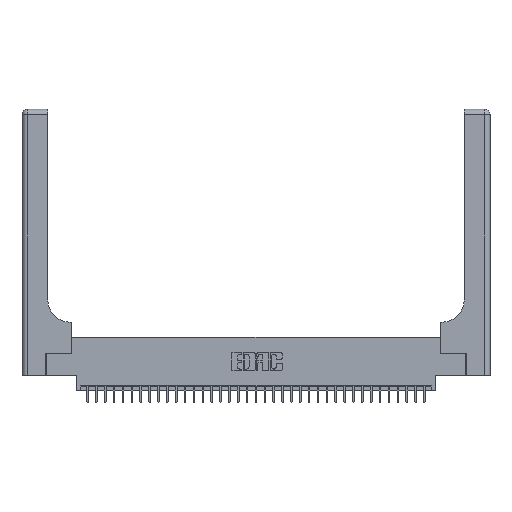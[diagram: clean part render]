
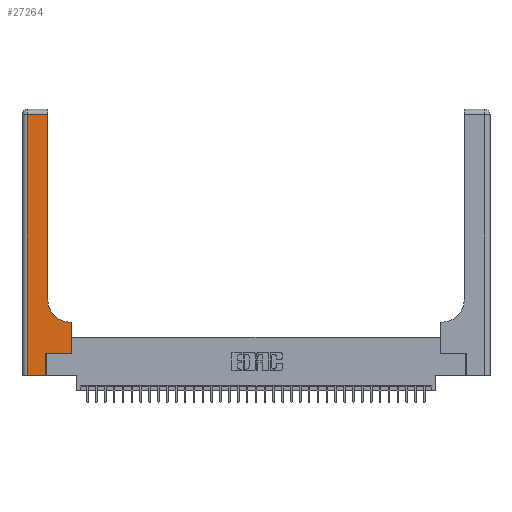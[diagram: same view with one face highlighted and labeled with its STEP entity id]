
A CAD part, top view. The second image highlights one B-rep face of the part: STEP entity #27264.
In plain terms, the highlighted planar face has unit normal (0, 0, 1).
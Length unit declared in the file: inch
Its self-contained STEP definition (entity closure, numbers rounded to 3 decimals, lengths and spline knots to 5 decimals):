
#1137 = ORIENTED_EDGE ( 'NONE', *, *, #33386, .T. ) ;
#1304 = DIRECTION ( 'NONE',  ( 0., 1., 0. ) ) ;
#1550 = ORIENTED_EDGE ( 'NONE', *, *, #27897, .T. ) ;
#2720 = CARTESIAN_POINT ( 'NONE',  ( 0.06, 3., 0.37 ) ) ;
#3202 = VERTEX_POINT ( 'NONE', #4219 ) ;
#3707 = DIRECTION ( 'NONE',  ( -1., 0., 0. ) ) ;
#4219 = CARTESIAN_POINT ( 'NONE',  ( 0.2915, 0.85, 0.37 ) ) ;
#4235 = LINE ( 'NONE', #32437, #14949 ) ;
#4299 = VECTOR ( 'NONE', #15855, 39.37008 ) ;
#4582 = CARTESIAN_POINT ( 'NONE',  ( 0., 3., 0.37 ) ) ;
#6160 = EDGE_LOOP ( 'NONE', ( #20468, #15500, #10927, #1550, #24159, #1137, #10253, #8115, #33073 ) ) ;
#6809 = PLANE ( 'NONE',  #35200 ) ;
#7383 = CARTESIAN_POINT ( 'NONE',  ( 0.269, 0., 0.37 ) ) ;
#8115 = ORIENTED_EDGE ( 'NONE', *, *, #22319, .T. ) ;
#8379 = DIRECTION ( 'NONE',  ( 1., 0., 0. ) ) ;
#8475 = VECTOR ( 'NONE', #31628, 39.37008 ) ;
#8681 = CARTESIAN_POINT ( 'NONE',  ( 0.2915, 3., 0.37 ) ) ;
#8790 = CARTESIAN_POINT ( 'NONE',  ( 0.2915, 0.6, 0.37 ) ) ;
#8953 = EDGE_CURVE ( 'NONE', #3202, #18350, #30642, .T. ) ;
#9272 = CARTESIAN_POINT ( 'NONE',  ( 0.269, 0.25, 0.37 ) ) ;
#9413 = CARTESIAN_POINT ( 'NONE',  ( 0., 0., 0.37 ) ) ;
#9962 = CARTESIAN_POINT ( 'NONE',  ( 0.5415, 0.6, 0.37 ) ) ;
#10114 = DIRECTION ( 'NONE',  ( 0., 0., -1. ) ) ;
#10167 = LINE ( 'NONE', #21413, #4299 ) ;
#10253 = ORIENTED_EDGE ( 'NONE', *, *, #17465, .T. ) ;
#10927 = ORIENTED_EDGE ( 'NONE', *, *, #33637, .T. ) ;
#11437 = CARTESIAN_POINT ( 'NONE',  ( 0., 2.94, 0.37 ) ) ;
#11893 = VERTEX_POINT ( 'NONE', #28991 ) ;
#12168 = LINE ( 'NONE', #9413, #22862 ) ;
#12413 = VERTEX_POINT ( 'NONE', #7383 ) ;
#13818 = VERTEX_POINT ( 'NONE', #9272 ) ;
#14084 = CIRCLE ( 'NONE', #21170, 0.25 ) ;
#14949 = VECTOR ( 'NONE', #18434, 39.37008 ) ;
#15500 = ORIENTED_EDGE ( 'NONE', *, *, #30966, .T. ) ;
#15843 = LINE ( 'NONE', #26585, #22836 ) ;
#15855 = DIRECTION ( 'NONE',  ( 0., 1., 0. ) ) ;
#16180 = DIRECTION ( 'NONE',  ( 0., -1., 0. ) ) ;
#16498 = VERTEX_POINT ( 'NONE', #25262 ) ;
#17465 = EDGE_CURVE ( 'NONE', #24648, #11893, #10167, .T. ) ;
#18051 = DIRECTION ( 'NONE',  ( -1., 0., 0. ) ) ;
#18350 = VERTEX_POINT ( 'NONE', #29979 ) ;
#18434 = DIRECTION ( 'NONE',  ( 1., 0., 0. ) ) ;
#20468 = ORIENTED_EDGE ( 'NONE', *, *, #8953, .T. ) ;
#20477 = LINE ( 'NONE', #11437, #22379 ) ;
#20573 = VECTOR ( 'NONE', #23054, 39.37008 ) ;
#21170 = AXIS2_PLACEMENT_3D ( 'NONE', #30857, #22396, #8379 ) ;
#21413 = CARTESIAN_POINT ( 'NONE',  ( 0.5585, 0.25, 0.37 ) ) ;
#22319 = EDGE_CURVE ( 'NONE', #11893, #28048, #28503, .T. ) ;
#22379 = VECTOR ( 'NONE', #3707, 39.37008 ) ;
#22396 = DIRECTION ( 'NONE',  ( 0., 0., -1. ) ) ;
#22836 = VECTOR ( 'NONE', #1304, 39.37008 ) ;
#22862 = VECTOR ( 'NONE', #28761, 39.37008 ) ;
#23054 = DIRECTION ( 'NONE',  ( 0., 1., 0. ) ) ;
#24159 = ORIENTED_EDGE ( 'NONE', *, *, #26855, .T. ) ;
#24648 = VERTEX_POINT ( 'NONE', #30681 ) ;
#25262 = CARTESIAN_POINT ( 'NONE',  ( 0.06, 2.94, 0.37 ) ) ;
#26367 = CARTESIAN_POINT ( 'NONE',  ( 0.06, 0., 0.37 ) ) ;
#26585 = CARTESIAN_POINT ( 'NONE',  ( 0.269, 0., 0.37 ) ) ;
#26855 = EDGE_CURVE ( 'NONE', #12413, #13818, #15843, .T. ) ;
#27264 = ADVANCED_FACE ( 'NONE', ( #29644 ), #6809, .F. ) ;
#27897 = EDGE_CURVE ( 'NONE', #33375, #12413, #12168, .T. ) ;
#27942 = VECTOR ( 'NONE', #16180, 39.37008 ) ;
#27990 = LINE ( 'NONE', #2720, #27942 ) ;
#28048 = VERTEX_POINT ( 'NONE', #9962 ) ;
#28503 = LINE ( 'NONE', #8790, #8475 ) ;
#28761 = DIRECTION ( 'NONE',  ( 1., 0., 0. ) ) ;
#28991 = CARTESIAN_POINT ( 'NONE',  ( 0.5585, 0.6, 0.37 ) ) ;
#29644 = FACE_OUTER_BOUND ( 'NONE', #6160, .T. ) ;
#29979 = CARTESIAN_POINT ( 'NONE',  ( 0.2915, 2.94, 0.37 ) ) ;
#30370 = EDGE_CURVE ( 'NONE', #28048, #3202, #14084, .T. ) ;
#30642 = LINE ( 'NONE', #8681, #20573 ) ;
#30681 = CARTESIAN_POINT ( 'NONE',  ( 0.5585, 0.25, 0.37 ) ) ;
#30857 = CARTESIAN_POINT ( 'NONE',  ( 0.5415, 0.85, 0.37 ) ) ;
#30966 = EDGE_CURVE ( 'NONE', #18350, #16498, #20477, .T. ) ;
#31628 = DIRECTION ( 'NONE',  ( -1., 0., 0. ) ) ;
#32437 = CARTESIAN_POINT ( 'NONE',  ( 0.269, 0.25, 0.37 ) ) ;
#33073 = ORIENTED_EDGE ( 'NONE', *, *, #30370, .T. ) ;
#33375 = VERTEX_POINT ( 'NONE', #26367 ) ;
#33386 = EDGE_CURVE ( 'NONE', #13818, #24648, #4235, .T. ) ;
#33637 = EDGE_CURVE ( 'NONE', #16498, #33375, #27990, .T. ) ;
#35200 = AXIS2_PLACEMENT_3D ( 'NONE', #4582, #10114, #18051 ) ;
